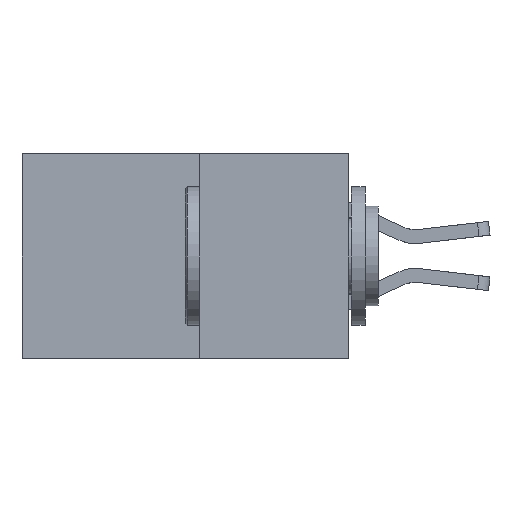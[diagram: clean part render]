
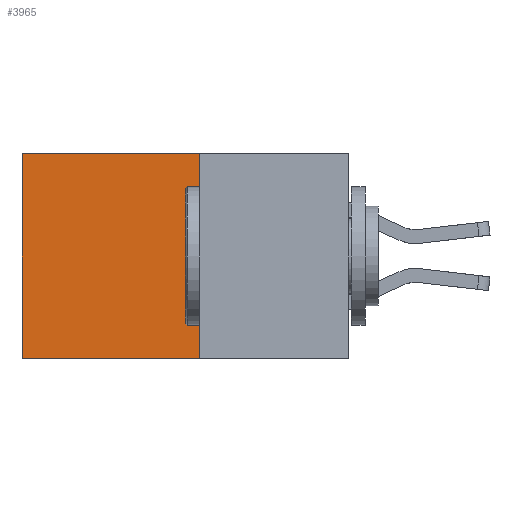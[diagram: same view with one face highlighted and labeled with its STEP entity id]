
A CAD part, left-side view. The second image highlights one B-rep face of the part: STEP entity #3965.
In plain terms, the highlighted planar face has unit normal (-1, 0, 0).
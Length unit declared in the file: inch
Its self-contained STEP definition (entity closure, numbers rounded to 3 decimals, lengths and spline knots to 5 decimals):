
#353 = CARTESIAN_POINT ( 'NONE',  ( 0.277, 0.59, 0. ) ) ;
#881 = CARTESIAN_POINT ( 'NONE',  ( 0.277, 0.27, -0.37 ) ) ;
#947 = ORIENTED_EDGE ( 'NONE', *, *, #3754, .F. ) ;
#1137 = EDGE_CURVE ( 'NONE', #10112, #10924, #10751, .T. ) ;
#1166 = VERTEX_POINT ( 'NONE', #353 ) ;
#1966 = DIRECTION ( 'NONE',  ( 0., 1., 0. ) ) ;
#2254 = VECTOR ( 'NONE', #4133, 39.37008 ) ;
#2258 = DIRECTION ( 'NONE',  ( 1., 0., 0. ) ) ;
#2281 = CARTESIAN_POINT ( 'NONE',  ( 0.277, 0.27, 0. ) ) ;
#2327 = CARTESIAN_POINT ( 'NONE',  ( 0.277, 0.27, -0.37 ) ) ;
#2374 = FACE_OUTER_BOUND ( 'NONE', #4972, .T. ) ;
#3005 = CARTESIAN_POINT ( 'NONE',  ( 0.277, 0.27, -0.37 ) ) ;
#3350 = CARTESIAN_POINT ( 'NONE',  ( 0.277, 0.27, 0. ) ) ;
#3399 = CARTESIAN_POINT ( 'NONE',  ( 0.277, 0.59, -0.37 ) ) ;
#3754 = EDGE_CURVE ( 'NONE', #4011, #10112, #6649, .T. ) ;
#3965 = ADVANCED_FACE ( 'NONE', ( #2374 ), #8659, .F. ) ;
#4011 = VERTEX_POINT ( 'NONE', #3350 ) ;
#4050 = DIRECTION ( 'NONE',  ( 0., 1., 0. ) ) ;
#4133 = DIRECTION ( 'NONE',  ( 0., 0., -1. ) ) ;
#4361 = VECTOR ( 'NONE', #1966, 39.37008 ) ;
#4693 = EDGE_CURVE ( 'NONE', #1166, #10924, #9418, .T. ) ;
#4845 = VECTOR ( 'NONE', #8393, 39.37008 ) ;
#4972 = EDGE_LOOP ( 'NONE', ( #7478, #6262, #947, #10287 ) ) ;
#5279 = LINE ( 'NONE', #2281, #6492 ) ;
#5425 = DIRECTION ( 'NONE',  ( 0., 0., -1. ) ) ;
#5630 = AXIS2_PLACEMENT_3D ( 'NONE', #881, #2258, #5425 ) ;
#6262 = ORIENTED_EDGE ( 'NONE', *, *, #1137, .F. ) ;
#6492 = VECTOR ( 'NONE', #4050, 39.37008 ) ;
#6649 = LINE ( 'NONE', #8205, #2254 ) ;
#7478 = ORIENTED_EDGE ( 'NONE', *, *, #4693, .T. ) ;
#8205 = CARTESIAN_POINT ( 'NONE',  ( 0.277, 0.27, -0.37 ) ) ;
#8393 = DIRECTION ( 'NONE',  ( 0., 0., -1. ) ) ;
#8597 = CARTESIAN_POINT ( 'NONE',  ( 0.277, 0.59, -0.37 ) ) ;
#8659 = PLANE ( 'NONE',  #5630 ) ;
#8994 = EDGE_CURVE ( 'NONE', #4011, #1166, #5279, .T. ) ;
#9418 = LINE ( 'NONE', #8597, #4845 ) ;
#10112 = VERTEX_POINT ( 'NONE', #3005 ) ;
#10287 = ORIENTED_EDGE ( 'NONE', *, *, #8994, .T. ) ;
#10751 = LINE ( 'NONE', #2327, #4361 ) ;
#10924 = VERTEX_POINT ( 'NONE', #3399 ) ;
